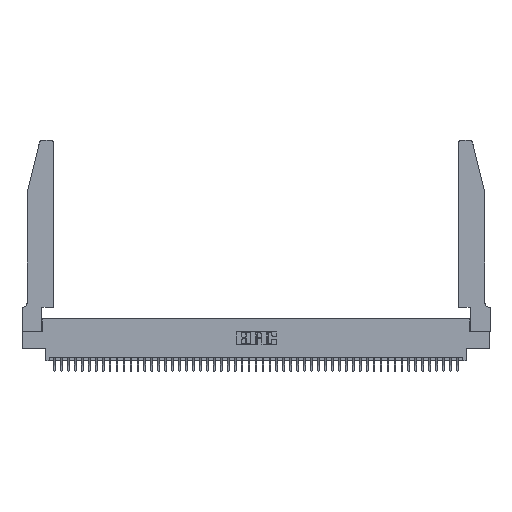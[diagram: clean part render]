
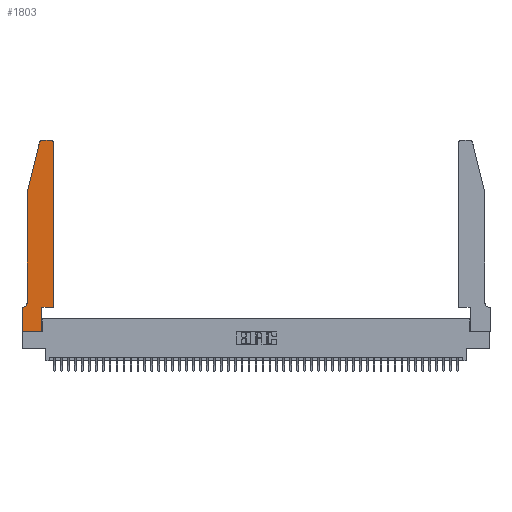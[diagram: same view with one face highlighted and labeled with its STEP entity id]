
A CAD part, top view. The second image highlights one B-rep face of the part: STEP entity #1803.
In plain terms, the highlighted planar face has unit normal (0, 0, 1).
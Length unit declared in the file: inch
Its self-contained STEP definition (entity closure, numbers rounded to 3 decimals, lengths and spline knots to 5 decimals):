
#1803 = ADVANCED_FACE ( 'NONE', ( #43622 ), #42179, .T. ) ;
#2084 = AXIS2_PLACEMENT_3D ( 'NONE', #11460, #6981, #22723 ) ;
#2773 = LINE ( 'NONE', #48300, #33002 ) ;
#2974 = DIRECTION ( 'NONE',  ( 1., 0., 0. ) ) ;
#3269 = CARTESIAN_POINT ( 'NONE',  ( 0., 0.35, 0.37 ) ) ;
#3355 = VERTEX_POINT ( 'NONE', #7751 ) ;
#3417 = EDGE_CURVE ( 'NONE', #47974, #30274, #6119, .T. ) ;
#3938 = CARTESIAN_POINT ( 'NONE',  ( 0.2605, 2.75, 0.37 ) ) ;
#4678 = EDGE_CURVE ( 'NONE', #30477, #40051, #41558, .T. ) ;
#4828 = DIRECTION ( 'NONE',  ( 1., 0., 0. ) ) ;
#5075 = CARTESIAN_POINT ( 'NONE',  ( 0.2865, 0.35, 0.37 ) ) ;
#5411 = LINE ( 'NONE', #47960, #18418 ) ;
#5953 = LINE ( 'NONE', #3938, #46895 ) ;
#6119 = CIRCLE ( 'NONE', #30358, 0.07 ) ;
#6178 = DIRECTION ( 'NONE',  ( 0., 0., 1. ) ) ;
#6845 = CARTESIAN_POINT ( 'NONE',  ( 0.4505, 0.35, 0.37 ) ) ;
#6981 = DIRECTION ( 'NONE',  ( 0., 0., 1. ) ) ;
#7743 = CARTESIAN_POINT ( 'NONE',  ( 0.0755, 2., 0.37 ) ) ;
#7751 = CARTESIAN_POINT ( 'NONE',  ( 0.4505, 2.72, 0.37 ) ) ;
#8487 = CARTESIAN_POINT ( 'NONE',  ( 0., 0.35, 0.37 ) ) ;
#11321 = CARTESIAN_POINT ( 'NONE',  ( 0.0755, 2., 0.37 ) ) ;
#11460 = CARTESIAN_POINT ( 'NONE',  ( 0.4205, 2.72, 0.37 ) ) ;
#11834 = VERTEX_POINT ( 'NONE', #39360 ) ;
#12179 = CARTESIAN_POINT ( 'NONE',  ( 0.25487, 2.72718, 0.37 ) ) ;
#12714 = LINE ( 'NONE', #6845, #15063 ) ;
#12923 = CARTESIAN_POINT ( 'NONE',  ( 0.2865, 0., 0.37 ) ) ;
#13073 = CIRCLE ( 'NONE', #2084, 0.03 ) ;
#13501 = CARTESIAN_POINT ( 'NONE',  ( 0., 0., 0.37 ) ) ;
#14687 = EDGE_CURVE ( 'NONE', #42569, #21649, #2773, .T. ) ;
#15063 = VECTOR ( 'NONE', #33344, 39.37008 ) ;
#15428 = CIRCLE ( 'NONE', #17574, 0.03 ) ;
#15459 = VECTOR ( 'NONE', #36192, 39.37008 ) ;
#16668 = EDGE_CURVE ( 'NONE', #35913, #3355, #47783, .T. ) ;
#17493 = ORIENTED_EDGE ( 'NONE', *, *, #14687, .T. ) ;
#17574 = AXIS2_PLACEMENT_3D ( 'NONE', #23017, #37934, #22516 ) ;
#18418 = VECTOR ( 'NONE', #2974, 39.37008 ) ;
#18506 = EDGE_CURVE ( 'NONE', #20868, #42569, #5411, .T. ) ;
#19059 = CARTESIAN_POINT ( 'NONE',  ( 0., 0., 0.37 ) ) ;
#20643 = CARTESIAN_POINT ( 'NONE',  ( 0.0055, 0.35, 0.37 ) ) ;
#20868 = VERTEX_POINT ( 'NONE', #19059 ) ;
#21649 = VERTEX_POINT ( 'NONE', #5075 ) ;
#21770 = VECTOR ( 'NONE', #26340, 39.37008 ) ;
#22174 = DIRECTION ( 'NONE',  ( -1., 0., 0. ) ) ;
#22354 = DIRECTION ( 'NONE',  ( 0., 0., -1. ) ) ;
#22486 = ORIENTED_EDGE ( 'NONE', *, *, #40306, .T. ) ;
#22506 = DIRECTION ( 'NONE',  ( 0., -1., 0. ) ) ;
#22516 = DIRECTION ( 'NONE',  ( 1., 0., 0. ) ) ;
#22583 = EDGE_CURVE ( 'NONE', #27088, #11834, #5953, .T. ) ;
#22723 = DIRECTION ( 'NONE',  ( 1., 0., 0. ) ) ;
#22766 = ORIENTED_EDGE ( 'NONE', *, *, #18506, .T. ) ;
#23015 = CARTESIAN_POINT ( 'NONE',  ( 0.0055, 0.42, 0.37 ) ) ;
#23017 = CARTESIAN_POINT ( 'NONE',  ( 0.284, 2.72, 0.37 ) ) ;
#23087 = DIRECTION ( 'NONE',  ( -0.239, -0.971, 0. ) ) ;
#24924 = AXIS2_PLACEMENT_3D ( 'NONE', #8487, #6178, #4828 ) ;
#25548 = LINE ( 'NONE', #13501, #15459 ) ;
#26177 = DIRECTION ( 'NONE',  ( -1., 0., 0. ) ) ;
#26340 = DIRECTION ( 'NONE',  ( -1., 0., 0. ) ) ;
#26359 = DIRECTION ( 'NONE',  ( 0., 1., 0. ) ) ;
#26508 = ORIENTED_EDGE ( 'NONE', *, *, #49027, .T. ) ;
#27088 = VERTEX_POINT ( 'NONE', #46425 ) ;
#27243 = CARTESIAN_POINT ( 'NONE',  ( 0.4505, 0.35, 0.37 ) ) ;
#28302 = ORIENTED_EDGE ( 'NONE', *, *, #16668, .T. ) ;
#29814 = DIRECTION ( 'NONE',  ( 0., 1., 0. ) ) ;
#30274 = VERTEX_POINT ( 'NONE', #20643 ) ;
#30358 = AXIS2_PLACEMENT_3D ( 'NONE', #23015, #22354, #26177 ) ;
#30477 = VERTEX_POINT ( 'NONE', #12179 ) ;
#31366 = ORIENTED_EDGE ( 'NONE', *, *, #48780, .T. ) ;
#31461 = EDGE_CURVE ( 'NONE', #21649, #35913, #12714, .T. ) ;
#31536 = CARTESIAN_POINT ( 'NONE',  ( 0.0755, 2., 0.37 ) ) ;
#32185 = EDGE_CURVE ( 'NONE', #30274, #38976, #48519, .T. ) ;
#33002 = VECTOR ( 'NONE', #26359, 39.37008 ) ;
#33344 = DIRECTION ( 'NONE',  ( 1., 0., 0. ) ) ;
#33777 = CARTESIAN_POINT ( 'NONE',  ( 0.0755, 0.35, 0.37 ) ) ;
#35185 = ORIENTED_EDGE ( 'NONE', *, *, #31461, .T. ) ;
#35516 = EDGE_LOOP ( 'NONE', ( #37333, #22486, #36498, #38198, #40062, #36329, #31366, #22766, #17493, #35185, #28302, #26508 ) ) ;
#35913 = VERTEX_POINT ( 'NONE', #27243 ) ;
#36192 = DIRECTION ( 'NONE',  ( 0., -1., 0. ) ) ;
#36329 = ORIENTED_EDGE ( 'NONE', *, *, #32185, .T. ) ;
#36498 = ORIENTED_EDGE ( 'NONE', *, *, #4678, .T. ) ;
#37091 = EDGE_CURVE ( 'NONE', #40051, #47974, #48678, .T. ) ;
#37333 = ORIENTED_EDGE ( 'NONE', *, *, #22583, .T. ) ;
#37637 = VECTOR ( 'NONE', #29814, 39.37008 ) ;
#37934 = DIRECTION ( 'NONE',  ( 0., 0., 1. ) ) ;
#38198 = ORIENTED_EDGE ( 'NONE', *, *, #37091, .T. ) ;
#38543 = VECTOR ( 'NONE', #22506, 39.37008 ) ;
#38976 = VERTEX_POINT ( 'NONE', #3269 ) ;
#39360 = CARTESIAN_POINT ( 'NONE',  ( 0.284, 2.75, 0.37 ) ) ;
#40051 = VERTEX_POINT ( 'NONE', #31536 ) ;
#40062 = ORIENTED_EDGE ( 'NONE', *, *, #3417, .T. ) ;
#40306 = EDGE_CURVE ( 'NONE', #11834, #30477, #15428, .T. ) ;
#41558 = LINE ( 'NONE', #11321, #48104 ) ;
#42179 = PLANE ( 'NONE',  #24924 ) ;
#42569 = VERTEX_POINT ( 'NONE', #12923 ) ;
#43622 = FACE_OUTER_BOUND ( 'NONE', #35516, .T. ) ;
#45607 = CARTESIAN_POINT ( 'NONE',  ( 0.4505, 0.35, 0.37 ) ) ;
#46425 = CARTESIAN_POINT ( 'NONE',  ( 0.4205, 2.75, 0.37 ) ) ;
#46895 = VECTOR ( 'NONE', #22174, 39.37008 ) ;
#47573 = CARTESIAN_POINT ( 'NONE',  ( 0.0755, 0.42, 0.37 ) ) ;
#47783 = LINE ( 'NONE', #45607, #37637 ) ;
#47960 = CARTESIAN_POINT ( 'NONE',  ( 0., 0., 0.37 ) ) ;
#47974 = VERTEX_POINT ( 'NONE', #47573 ) ;
#48104 = VECTOR ( 'NONE', #23087, 39.37008 ) ;
#48300 = CARTESIAN_POINT ( 'NONE',  ( 0.2865, 0.35, 0.37 ) ) ;
#48519 = LINE ( 'NONE', #33777, #21770 ) ;
#48678 = LINE ( 'NONE', #7743, #38543 ) ;
#48780 = EDGE_CURVE ( 'NONE', #38976, #20868, #25548, .T. ) ;
#49027 = EDGE_CURVE ( 'NONE', #3355, #27088, #13073, .T. ) ;
